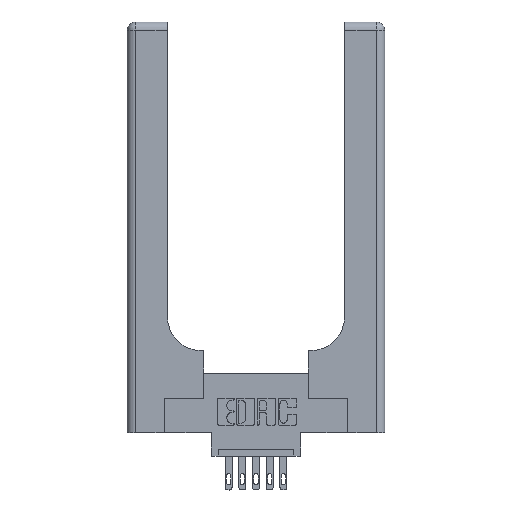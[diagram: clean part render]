
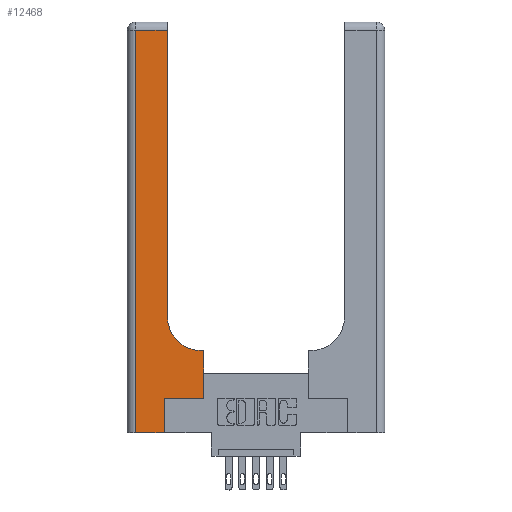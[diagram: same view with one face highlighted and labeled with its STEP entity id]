
A CAD part, top view. The second image highlights one B-rep face of the part: STEP entity #12468.
In plain terms, the highlighted planar face has unit normal (0, 0, 1).
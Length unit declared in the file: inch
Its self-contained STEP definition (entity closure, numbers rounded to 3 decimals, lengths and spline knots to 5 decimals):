
#264 = LINE ( 'NONE', #13220, #8167 ) ;
#324 = VECTOR ( 'NONE', #3140, 39.37008 ) ;
#846 = VERTEX_POINT ( 'NONE', #2019 ) ;
#1042 = DIRECTION ( 'NONE',  ( -1., 0., 0. ) ) ;
#1179 = ORIENTED_EDGE ( 'NONE', *, *, #8320, .T. ) ;
#1599 = VERTEX_POINT ( 'NONE', #8907 ) ;
#2019 = CARTESIAN_POINT ( 'NONE',  ( 0.269, 0., 0.37 ) ) ;
#2102 = PLANE ( 'NONE',  #5033 ) ;
#2251 = CARTESIAN_POINT ( 'NONE',  ( 0.2915, 3., 0.37 ) ) ;
#2352 = CIRCLE ( 'NONE', #9317, 0.25 ) ;
#2426 = DIRECTION ( 'NONE',  ( 0., 0., -1. ) ) ;
#2821 = ORIENTED_EDGE ( 'NONE', *, *, #6383, .T. ) ;
#2892 = ORIENTED_EDGE ( 'NONE', *, *, #6161, .T. ) ;
#2928 = CARTESIAN_POINT ( 'NONE',  ( 0., 3., 0.37 ) ) ;
#2943 = DIRECTION ( 'NONE',  ( 0., 1., 0. ) ) ;
#3140 = DIRECTION ( 'NONE',  ( 1., 0., 0. ) ) ;
#3365 = EDGE_CURVE ( 'NONE', #4276, #9095, #2352, .T. ) ;
#3605 = CARTESIAN_POINT ( 'NONE',  ( 0.2915, 0.85, 0.37 ) ) ;
#3615 = CARTESIAN_POINT ( 'NONE',  ( 0., 2.94, 0.37 ) ) ;
#3934 = EDGE_CURVE ( 'NONE', #10041, #4276, #4700, .T. ) ;
#4001 = CARTESIAN_POINT ( 'NONE',  ( 0.5585, 0.25, 0.37 ) ) ;
#4064 = VERTEX_POINT ( 'NONE', #4524 ) ;
#4246 = CARTESIAN_POINT ( 'NONE',  ( 0.269, 0., 0.37 ) ) ;
#4262 = LINE ( 'NONE', #4246, #12556 ) ;
#4276 = VERTEX_POINT ( 'NONE', #11714 ) ;
#4299 = CARTESIAN_POINT ( 'NONE',  ( 0.2915, 2.94, 0.37 ) ) ;
#4459 = LINE ( 'NONE', #3615, #12418 ) ;
#4471 = LINE ( 'NONE', #2251, #9874 ) ;
#4524 = CARTESIAN_POINT ( 'NONE',  ( 0.06, 0., 0.37 ) ) ;
#4566 = DIRECTION ( 'NONE',  ( -1., 0., 0. ) ) ;
#4641 = DIRECTION ( 'NONE',  ( 1., 0., 0. ) ) ;
#4700 = LINE ( 'NONE', #11744, #8585 ) ;
#4809 = LINE ( 'NONE', #4001, #7520 ) ;
#4992 = EDGE_LOOP ( 'NONE', ( #2821, #9623, #10668, #7501, #6773, #1179, #2892, #13599, #9028 ) ) ;
#5033 = AXIS2_PLACEMENT_3D ( 'NONE', #2928, #6206, #5388 ) ;
#5388 = DIRECTION ( 'NONE',  ( -1., 0., 0. ) ) ;
#5443 = FACE_OUTER_BOUND ( 'NONE', #4992, .T. ) ;
#5670 = CARTESIAN_POINT ( 'NONE',  ( 0.5585, 0.6, 0.37 ) ) ;
#5877 = LINE ( 'NONE', #10558, #324 ) ;
#5893 = EDGE_CURVE ( 'NONE', #1599, #4064, #6344, .T. ) ;
#6161 = EDGE_CURVE ( 'NONE', #6555, #10041, #4809, .T. ) ;
#6206 = DIRECTION ( 'NONE',  ( 0., 0., -1. ) ) ;
#6344 = LINE ( 'NONE', #9529, #8033 ) ;
#6383 = EDGE_CURVE ( 'NONE', #9095, #11496, #4471, .T. ) ;
#6555 = VERTEX_POINT ( 'NONE', #12096 ) ;
#6773 = ORIENTED_EDGE ( 'NONE', *, *, #11595, .T. ) ;
#6889 = DIRECTION ( 'NONE',  ( 1., 0., 0. ) ) ;
#7079 = EDGE_CURVE ( 'NONE', #11496, #1599, #4459, .T. ) ;
#7501 = ORIENTED_EDGE ( 'NONE', *, *, #11150, .T. ) ;
#7520 = VECTOR ( 'NONE', #2943, 39.37008 ) ;
#7790 = VERTEX_POINT ( 'NONE', #12068 ) ;
#8033 = VECTOR ( 'NONE', #13192, 39.37008 ) ;
#8167 = VECTOR ( 'NONE', #4641, 39.37008 ) ;
#8320 = EDGE_CURVE ( 'NONE', #7790, #6555, #5877, .T. ) ;
#8547 = DIRECTION ( 'NONE',  ( 0., 1., 0. ) ) ;
#8580 = DIRECTION ( 'NONE',  ( 0., 1., 0. ) ) ;
#8585 = VECTOR ( 'NONE', #1042, 39.37008 ) ;
#8907 = CARTESIAN_POINT ( 'NONE',  ( 0.06, 2.94, 0.37 ) ) ;
#9028 = ORIENTED_EDGE ( 'NONE', *, *, #3365, .T. ) ;
#9095 = VERTEX_POINT ( 'NONE', #3605 ) ;
#9317 = AXIS2_PLACEMENT_3D ( 'NONE', #13319, #2426, #6889 ) ;
#9529 = CARTESIAN_POINT ( 'NONE',  ( 0.06, 3., 0.37 ) ) ;
#9623 = ORIENTED_EDGE ( 'NONE', *, *, #7079, .T. ) ;
#9874 = VECTOR ( 'NONE', #8580, 39.37008 ) ;
#10041 = VERTEX_POINT ( 'NONE', #5670 ) ;
#10558 = CARTESIAN_POINT ( 'NONE',  ( 0.269, 0.25, 0.37 ) ) ;
#10668 = ORIENTED_EDGE ( 'NONE', *, *, #5893, .T. ) ;
#11150 = EDGE_CURVE ( 'NONE', #4064, #846, #264, .T. ) ;
#11496 = VERTEX_POINT ( 'NONE', #4299 ) ;
#11595 = EDGE_CURVE ( 'NONE', #846, #7790, #4262, .T. ) ;
#11714 = CARTESIAN_POINT ( 'NONE',  ( 0.5415, 0.6, 0.37 ) ) ;
#11744 = CARTESIAN_POINT ( 'NONE',  ( 0.2915, 0.6, 0.37 ) ) ;
#12068 = CARTESIAN_POINT ( 'NONE',  ( 0.269, 0.25, 0.37 ) ) ;
#12096 = CARTESIAN_POINT ( 'NONE',  ( 0.5585, 0.25, 0.37 ) ) ;
#12418 = VECTOR ( 'NONE', #4566, 39.37008 ) ;
#12468 = ADVANCED_FACE ( 'NONE', ( #5443 ), #2102, .F. ) ;
#12556 = VECTOR ( 'NONE', #8547, 39.37008 ) ;
#13192 = DIRECTION ( 'NONE',  ( 0., -1., 0. ) ) ;
#13220 = CARTESIAN_POINT ( 'NONE',  ( 0., 0., 0.37 ) ) ;
#13319 = CARTESIAN_POINT ( 'NONE',  ( 0.5415, 0.85, 0.37 ) ) ;
#13599 = ORIENTED_EDGE ( 'NONE', *, *, #3934, .T. ) ;
